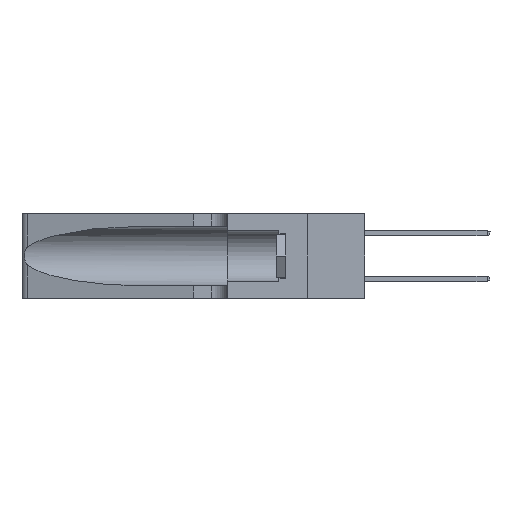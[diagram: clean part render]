
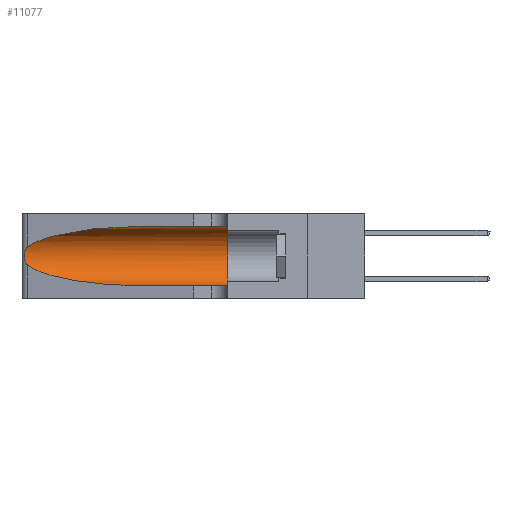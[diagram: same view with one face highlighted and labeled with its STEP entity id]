
A CAD part, left-side view. The second image highlights one B-rep face of the part: STEP entity #11077.
In plain terms, the highlighted cylindrical face has radius 3.308 mm (diameter 6.617 mm), a partial arc.
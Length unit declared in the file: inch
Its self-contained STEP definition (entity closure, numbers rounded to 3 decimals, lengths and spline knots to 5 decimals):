
#319 = CARTESIAN_POINT ( 'NONE',  ( 0.25487, 1.22718, 0.22369 ) ) ;
#761 = CARTESIAN_POINT ( 'NONE',  ( 0.2373, 1.15595, 0.28018 ) ) ;
#853 = VERTEX_POINT ( 'NONE', #28147 ) ;
#1272 = ORIENTED_EDGE ( 'NONE', *, *, #20952, .F. ) ;
#1851 = CARTESIAN_POINT ( 'NONE',  ( 0.25639, 1.23184, 0.21858 ) ) ;
#2030 = CARTESIAN_POINT ( 'NONE',  ( 0.1305, 0.72297, 0.05475 ) ) ;
#2079 = CARTESIAN_POINT ( 'NONE',  ( 0.25639, 1.23186, 0.15144 ) ) ;
#2238 = CARTESIAN_POINT ( 'NONE',  ( 0.1305, 1.61858, 0.185 ) ) ;
#2458 = DIRECTION ( 'NONE',  ( 0., -1., 0. ) ) ;
#2552 = VERTEX_POINT ( 'NONE', #7332 ) ;
#2749 = VERTEX_POINT ( 'NONE', #4531 ) ;
#3117 = VECTOR ( 'NONE', #31787, 39.37008 ) ;
#3380 = EDGE_CURVE ( 'NONE', #28493, #2749, #8885, .T. ) ;
#3494 = CYLINDRICAL_SURFACE ( 'NONE', #32118, 0.13025 ) ;
#3787 = DIRECTION ( 'NONE',  ( 0., 0., 1. ) ) ;
#4347 = CARTESIAN_POINT ( 'NONE',  ( 0.25789, 1.23486, 0.15765 ) ) ;
#4531 = CARTESIAN_POINT ( 'NONE',  ( 0.25487, 1.22718, 0.22369 ) ) ;
#4970 = DIRECTION ( 'NONE',  ( 0., 0., -1. ) ) ;
#5463 = VECTOR ( 'NONE', #22916, 39.37008 ) ;
#5867 = EDGE_CURVE ( 'NONE', #32746, #2552, #21112, .T. ) ;
#6537 = ORIENTED_EDGE ( 'NONE', *, *, #3380, .T. ) ;
#6665 = CARTESIAN_POINT ( 'NONE',  ( 0.1305, 0.72297, 0.31525 ) ) ;
#7332 = CARTESIAN_POINT ( 'NONE',  ( 0.1305, 0.35, 0.05475 ) ) ;
#8885 =( BOUNDED_CURVE ( )  B_SPLINE_CURVE ( 3, ( #27578, #12669, #761, #319 ),
 .UNSPECIFIED., .F., .F. ) 
 B_SPLINE_CURVE_WITH_KNOTS ( ( 4, 4 ),
 ( 1.5708, 2.84003 ),
 .UNSPECIFIED. ) 
 CURVE ( )  GEOMETRIC_REPRESENTATION_ITEM ( )  RATIONAL_B_SPLINE_CURVE ( ( 1., 0.87, 0.87, 1. ) ) 
 REPRESENTATION_ITEM ( '' )  );
#9489 = CARTESIAN_POINT ( 'NONE',  ( 0.26017, 1.23833, 0.17102 ) ) ;
#10338 = CIRCLE ( 'NONE', #31281, 0.13025 ) ;
#11077 = ADVANCED_FACE ( 'NONE', ( #25520 ), #3494, .F. ) ;
#11956 = ORIENTED_EDGE ( 'NONE', *, *, #14482, .T. ) ;
#11969 = CARTESIAN_POINT ( 'NONE',  ( 0.25787, 1.23484, 0.2124 ) ) ;
#12069 = CARTESIAN_POINT ( 'NONE',  ( 0.25487, 1.22718, 0.14631 ) ) ;
#12197 = CARTESIAN_POINT ( 'NONE',  ( 0.25487, 1.22718, 0.22369 ) ) ;
#12669 = CARTESIAN_POINT ( 'NONE',  ( 0.18966, 0.96281, 0.31525 ) ) ;
#12776 = CARTESIAN_POINT ( 'NONE',  ( 0.18966, 0.96281, 0.05475 ) ) ;
#13858 = CARTESIAN_POINT ( 'NONE',  ( 0.1305, 1.61858, 0.31525 ) ) ;
#13961 = VERTEX_POINT ( 'NONE', #23312 ) ;
#14379 = CARTESIAN_POINT ( 'NONE',  ( 0.26018, 1.23835, 0.19895 ) ) ;
#14482 = EDGE_CURVE ( 'NONE', #2749, #853, #31209, .T. ) ;
#14500 = CARTESIAN_POINT ( 'NONE',  ( 0.26075, 1.23896, 0.178 ) ) ;
#14614 = CARTESIAN_POINT ( 'NONE',  ( 0.26075, 1.23896, 0.19203 ) ) ;
#20415 = CARTESIAN_POINT ( 'NONE',  ( 0.1305, 0.72297, 0.05475 ) ) ;
#20716 =( BOUNDED_CURVE ( )  B_SPLINE_CURVE ( 3, ( #25349, #28148, #12776, #20415 ),
 .UNSPECIFIED., .F., .T. ) 
 B_SPLINE_CURVE_WITH_KNOTS ( ( 4, 4 ),
 ( 3.44316, 4.71239 ),
 .UNSPECIFIED. ) 
 CURVE ( )  GEOMETRIC_REPRESENTATION_ITEM ( )  RATIONAL_B_SPLINE_CURVE ( ( 1., 0.87, 0.87, 1. ) ) 
 REPRESENTATION_ITEM ( '' )  );
#20952 = EDGE_CURVE ( 'NONE', #28493, #13961, #28344, .T. ) ;
#21112 = LINE ( 'NONE', #31027, #5463 ) ;
#21950 = CARTESIAN_POINT ( 'NONE',  ( 0.1305, 0.35, 0.185 ) ) ;
#22284 = CARTESIAN_POINT ( 'NONE',  ( 0.25555, 1.22993, 0.14849 ) ) ;
#22916 = DIRECTION ( 'NONE',  ( 0., -1., 0. ) ) ;
#23312 = CARTESIAN_POINT ( 'NONE',  ( 0.1305, 0.35, 0.31525 ) ) ;
#25349 = CARTESIAN_POINT ( 'NONE',  ( 0.25487, 1.22718, 0.14631 ) ) ;
#25483 = EDGE_CURVE ( 'NONE', #13961, #2552, #10338, .T. ) ;
#25520 = FACE_OUTER_BOUND ( 'NONE', #29541, .T. ) ;
#25939 = EDGE_CURVE ( 'NONE', #853, #32746, #20716, .T. ) ;
#26183 = ORIENTED_EDGE ( 'NONE', *, *, #25483, .F. ) ;
#27566 = CARTESIAN_POINT ( 'NONE',  ( 0.25854, 1.2359, 0.20912 ) ) ;
#27578 = CARTESIAN_POINT ( 'NONE',  ( 0.1305, 0.72297, 0.31525 ) ) ;
#28147 = CARTESIAN_POINT ( 'NONE',  ( 0.25487, 1.22718, 0.14631 ) ) ;
#28148 = CARTESIAN_POINT ( 'NONE',  ( 0.2373, 1.15595, 0.08982 ) ) ;
#28344 = LINE ( 'NONE', #13858, #3117 ) ;
#28493 = VERTEX_POINT ( 'NONE', #6665 ) ;
#29541 = EDGE_LOOP ( 'NONE', ( #6537, #11956, #29834, #31895, #26183, #1272 ) ) ;
#29834 = ORIENTED_EDGE ( 'NONE', *, *, #25939, .T. ) ;
#31027 = CARTESIAN_POINT ( 'NONE',  ( 0.1305, 1.61858, 0.05475 ) ) ;
#31209 = B_SPLINE_CURVE_WITH_KNOTS ( 'NONE', 3,
 ( #12197, #32547, #1851, #11969, #27566, #14379, #14614, #14500, #9489, #32317, #4347, #2079, #22284, #12069 ),
 .UNSPECIFIED., .F., .F.,
 ( 4, 2, 2, 2, 2, 2, 4 ),
 ( 0., 0.00027, 0.00053, 0.00107, 0.0016, 0.00187, 0.00214 ),
 .UNSPECIFIED. ) ;
#31281 = AXIS2_PLACEMENT_3D ( 'NONE', #21950, #32109, #3787 ) ;
#31787 = DIRECTION ( 'NONE',  ( 0., -1., 0. ) ) ;
#31895 = ORIENTED_EDGE ( 'NONE', *, *, #5867, .T. ) ;
#32109 = DIRECTION ( 'NONE',  ( 0., 1., 0. ) ) ;
#32118 = AXIS2_PLACEMENT_3D ( 'NONE', #2238, #2458, #4970 ) ;
#32317 = CARTESIAN_POINT ( 'NONE',  ( 0.25856, 1.23593, 0.16098 ) ) ;
#32547 = CARTESIAN_POINT ( 'NONE',  ( 0.25555, 1.22994, 0.2215 ) ) ;
#32746 = VERTEX_POINT ( 'NONE', #2030 ) ;
